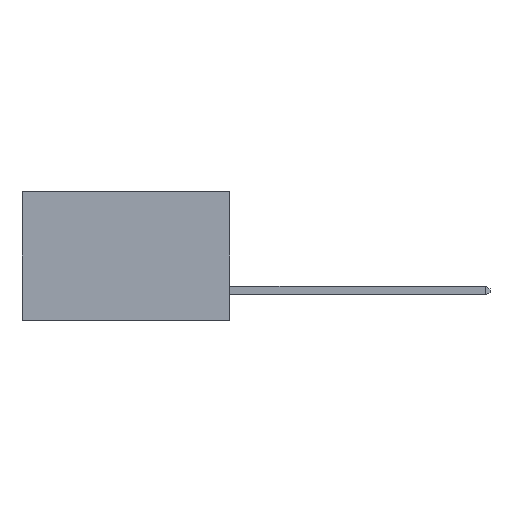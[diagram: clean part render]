
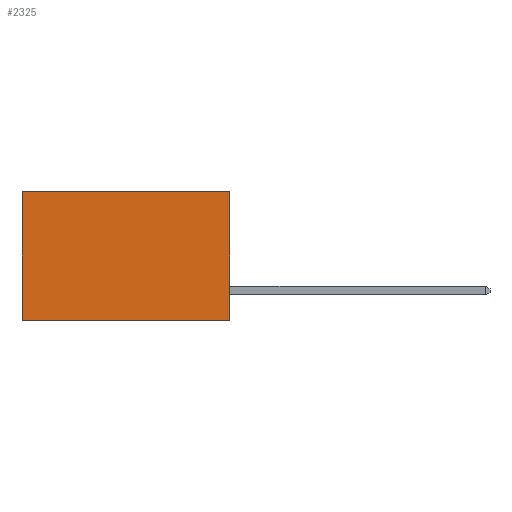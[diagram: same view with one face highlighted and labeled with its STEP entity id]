
A CAD part, left-side view. The second image highlights one B-rep face of the part: STEP entity #2325.
In plain terms, the highlighted planar face has unit normal (-1, 0, 0).
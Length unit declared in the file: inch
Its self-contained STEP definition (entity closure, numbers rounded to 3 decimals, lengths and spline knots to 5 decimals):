
#2155 = CARTESIAN_POINT ( 'NONE',  ( 0.298, 0.6, 0. ) ) ;
#2240 = EDGE_CURVE ( 'NONE', #10962, #12633, #8757, .T. ) ;
#2325 = ADVANCED_FACE ( 'NONE', ( #9796 ), #5964, .F. ) ;
#3113 = ORIENTED_EDGE ( 'NONE', *, *, #12304, .T. ) ;
#3168 = VERTEX_POINT ( 'NONE', #2155 ) ;
#3183 = ORIENTED_EDGE ( 'NONE', *, *, #6758, .F. ) ;
#3211 = AXIS2_PLACEMENT_3D ( 'NONE', #4074, #9676, #12726 ) ;
#3217 = ORIENTED_EDGE ( 'NONE', *, *, #2240, .F. ) ;
#3268 = DIRECTION ( 'NONE',  ( 0., 0., -1. ) ) ;
#3532 = ORIENTED_EDGE ( 'NONE', *, *, #10206, .T. ) ;
#3680 = VECTOR ( 'NONE', #3268, 39.37008 ) ;
#4074 = CARTESIAN_POINT ( 'NONE',  ( 0.298, 0., 0. ) ) ;
#5143 = CARTESIAN_POINT ( 'NONE',  ( 0.298, 0., 0. ) ) ;
#5964 = PLANE ( 'NONE',  #3211 ) ;
#6233 = LINE ( 'NONE', #12199, #8854 ) ;
#6307 = VERTEX_POINT ( 'NONE', #8246 ) ;
#6318 = LINE ( 'NONE', #10662, #8614 ) ;
#6758 = EDGE_CURVE ( 'NONE', #12633, #6307, #6318, .T. ) ;
#7064 = LINE ( 'NONE', #5143, #9319 ) ;
#7146 = CARTESIAN_POINT ( 'NONE',  ( 0.298, 0., 0. ) ) ;
#8145 = DIRECTION ( 'NONE',  ( 0., 1., 0. ) ) ;
#8246 = CARTESIAN_POINT ( 'NONE',  ( 0.298, 0.6, -0.37 ) ) ;
#8369 = EDGE_LOOP ( 'NONE', ( #3113, #3183, #3217, #3532 ) ) ;
#8614 = VECTOR ( 'NONE', #10502, 39.37008 ) ;
#8757 = LINE ( 'NONE', #7146, #3680 ) ;
#8854 = VECTOR ( 'NONE', #10456, 39.37008 ) ;
#9319 = VECTOR ( 'NONE', #8145, 39.37008 ) ;
#9676 = DIRECTION ( 'NONE',  ( 1., 0., 0. ) ) ;
#9796 = FACE_OUTER_BOUND ( 'NONE', #8369, .T. ) ;
#9950 = CARTESIAN_POINT ( 'NONE',  ( 0.298, 0., 0. ) ) ;
#10206 = EDGE_CURVE ( 'NONE', #10962, #3168, #7064, .T. ) ;
#10456 = DIRECTION ( 'NONE',  ( 0., 0., -1. ) ) ;
#10502 = DIRECTION ( 'NONE',  ( 0., 1., 0. ) ) ;
#10662 = CARTESIAN_POINT ( 'NONE',  ( 0.298, 0., -0.37 ) ) ;
#10775 = CARTESIAN_POINT ( 'NONE',  ( 0.298, 0., -0.37 ) ) ;
#10962 = VERTEX_POINT ( 'NONE', #9950 ) ;
#12199 = CARTESIAN_POINT ( 'NONE',  ( 0.298, 0.6, 0. ) ) ;
#12304 = EDGE_CURVE ( 'NONE', #3168, #6307, #6233, .T. ) ;
#12633 = VERTEX_POINT ( 'NONE', #10775 ) ;
#12726 = DIRECTION ( 'NONE',  ( 0., 0., -1. ) ) ;
